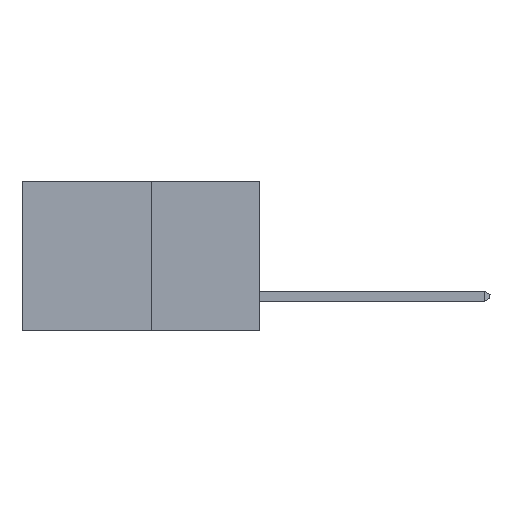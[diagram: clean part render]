
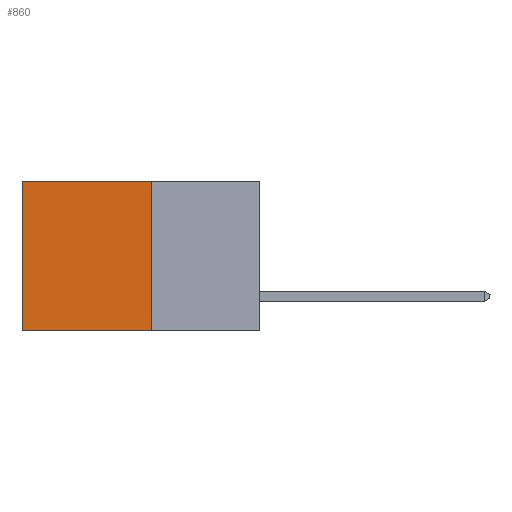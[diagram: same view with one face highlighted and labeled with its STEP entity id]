
A CAD part, left-side view. The second image highlights one B-rep face of the part: STEP entity #860.
In plain terms, the highlighted planar face has unit normal (-1, 0, 0).
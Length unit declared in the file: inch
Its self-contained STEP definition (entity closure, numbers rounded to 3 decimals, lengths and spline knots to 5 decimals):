
#151 = DIRECTION ( 'NONE',  ( 0., 0., -1. ) ) ;
#355 = VECTOR ( 'NONE', #7783, 39.37008 ) ;
#860 = ADVANCED_FACE ( 'NONE', ( #5214 ), #5526, .F. ) ;
#1256 = EDGE_CURVE ( 'NONE', #1929, #4245, #8169, .T. ) ;
#1929 = VERTEX_POINT ( 'NONE', #3664 ) ;
#2838 = CARTESIAN_POINT ( 'NONE',  ( 0.277, 0.27, 0. ) ) ;
#3371 = VECTOR ( 'NONE', #9114, 39.37008 ) ;
#3525 = ORIENTED_EDGE ( 'NONE', *, *, #7993, .T. ) ;
#3664 = CARTESIAN_POINT ( 'NONE',  ( 0.277, 0.27, -0.37 ) ) ;
#4142 = CARTESIAN_POINT ( 'NONE',  ( 0.277, 0.59, -0.37 ) ) ;
#4245 = VERTEX_POINT ( 'NONE', #8954 ) ;
#4814 = DIRECTION ( 'NONE',  ( 0., 0., -1. ) ) ;
#4826 = DIRECTION ( 'NONE',  ( 1., 0., 0. ) ) ;
#5214 = FACE_OUTER_BOUND ( 'NONE', #7220, .T. ) ;
#5218 = VECTOR ( 'NONE', #5916, 39.37008 ) ;
#5313 = CARTESIAN_POINT ( 'NONE',  ( 0.277, 0.27, -0.37 ) ) ;
#5419 = CARTESIAN_POINT ( 'NONE',  ( 0.277, 0.27, -0.37 ) ) ;
#5526 = PLANE ( 'NONE',  #6266 ) ;
#5916 = DIRECTION ( 'NONE',  ( 0., 1., 0. ) ) ;
#6087 = EDGE_CURVE ( 'NONE', #10778, #10975, #7863, .T. ) ;
#6120 = ORIENTED_EDGE ( 'NONE', *, *, #6087, .T. ) ;
#6266 = AXIS2_PLACEMENT_3D ( 'NONE', #5419, #4826, #4814 ) ;
#6947 = CARTESIAN_POINT ( 'NONE',  ( 0.277, 0.59, 0. ) ) ;
#7220 = EDGE_LOOP ( 'NONE', ( #3525, #12793, #11368, #6120 ) ) ;
#7766 = CARTESIAN_POINT ( 'NONE',  ( 0.277, 0.27, -0.37 ) ) ;
#7783 = DIRECTION ( 'NONE',  ( 0., 1., 0. ) ) ;
#7863 = LINE ( 'NONE', #2838, #5218 ) ;
#7993 = EDGE_CURVE ( 'NONE', #10975, #4245, #8705, .T. ) ;
#8169 = LINE ( 'NONE', #7766, #355 ) ;
#8705 = LINE ( 'NONE', #4142, #3371 ) ;
#8954 = CARTESIAN_POINT ( 'NONE',  ( 0.277, 0.59, -0.37 ) ) ;
#9114 = DIRECTION ( 'NONE',  ( 0., 0., -1. ) ) ;
#9778 = LINE ( 'NONE', #5313, #12460 ) ;
#10562 = CARTESIAN_POINT ( 'NONE',  ( 0.277, 0.27, 0. ) ) ;
#10778 = VERTEX_POINT ( 'NONE', #10562 ) ;
#10975 = VERTEX_POINT ( 'NONE', #6947 ) ;
#11368 = ORIENTED_EDGE ( 'NONE', *, *, #12327, .F. ) ;
#12327 = EDGE_CURVE ( 'NONE', #10778, #1929, #9778, .T. ) ;
#12460 = VECTOR ( 'NONE', #151, 39.37008 ) ;
#12793 = ORIENTED_EDGE ( 'NONE', *, *, #1256, .F. ) ;
